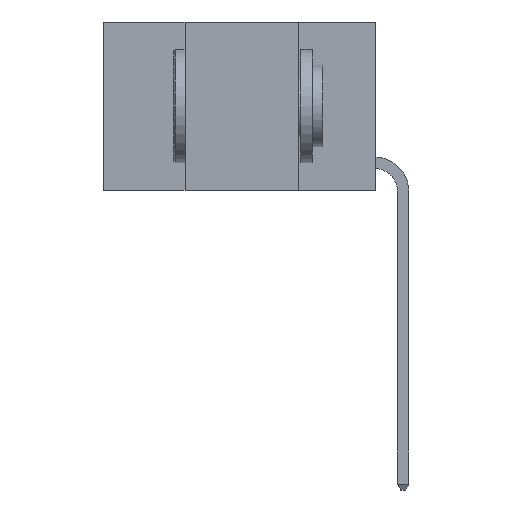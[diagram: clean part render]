
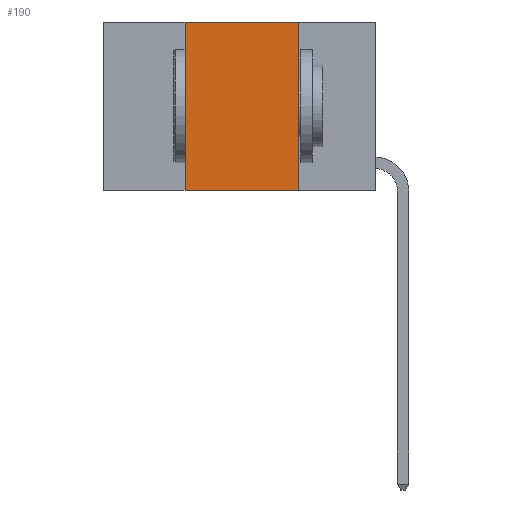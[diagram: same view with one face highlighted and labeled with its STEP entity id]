
A CAD part, left-side view. The second image highlights one B-rep face of the part: STEP entity #190.
In plain terms, the highlighted planar face has unit normal (-1, 0, 0).
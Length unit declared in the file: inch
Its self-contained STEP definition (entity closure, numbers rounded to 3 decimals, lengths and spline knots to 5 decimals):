
#190 = ADVANCED_FACE ( 'NONE', ( #4583 ), #807, .F. ) ;
#435 = CARTESIAN_POINT ( 'NONE',  ( 0., 0.42, -0.37 ) ) ;
#551 = ORIENTED_EDGE ( 'NONE', *, *, #1379, .F. ) ;
#807 = PLANE ( 'NONE',  #5528 ) ;
#838 = ORIENTED_EDGE ( 'NONE', *, *, #8155, .F. ) ;
#1355 = LINE ( 'NONE', #10478, #5852 ) ;
#1379 = EDGE_CURVE ( 'NONE', #9485, #5882, #5469, .T. ) ;
#1880 = CARTESIAN_POINT ( 'NONE',  ( 0., 0.6, 0. ) ) ;
#1991 = EDGE_CURVE ( 'NONE', #10167, #2492, #1355, .T. ) ;
#2492 = VERTEX_POINT ( 'NONE', #7672 ) ;
#3463 = DIRECTION ( 'NONE',  ( 0., 0., 1. ) ) ;
#4343 = DIRECTION ( 'NONE',  ( 0., 0., -1. ) ) ;
#4521 = ORIENTED_EDGE ( 'NONE', *, *, #6401, .T. ) ;
#4583 = FACE_OUTER_BOUND ( 'NONE', #9444, .T. ) ;
#5197 = CARTESIAN_POINT ( 'NONE',  ( 0., 0.42, 0. ) ) ;
#5469 = LINE ( 'NONE', #5197, #9484 ) ;
#5505 = LINE ( 'NONE', #11246, #7529 ) ;
#5528 = AXIS2_PLACEMENT_3D ( 'NONE', #5566, #11139, #4343 ) ;
#5566 = CARTESIAN_POINT ( 'NONE',  ( 0., 0.6, 0. ) ) ;
#5852 = VECTOR ( 'NONE', #6201, 39.37008 ) ;
#5869 = LINE ( 'NONE', #1880, #8170 ) ;
#5882 = VERTEX_POINT ( 'NONE', #8837 ) ;
#6107 = DIRECTION ( 'NONE',  ( 0., -1., 0. ) ) ;
#6201 = DIRECTION ( 'NONE',  ( 0., 0., -1. ) ) ;
#6401 = EDGE_CURVE ( 'NONE', #9485, #2492, #5505, .T. ) ;
#7529 = VECTOR ( 'NONE', #6107, 39.37008 ) ;
#7672 = CARTESIAN_POINT ( 'NONE',  ( 0., 0.17, -0.37 ) ) ;
#8155 = EDGE_CURVE ( 'NONE', #5882, #10167, #5869, .T. ) ;
#8170 = VECTOR ( 'NONE', #8928, 39.37008 ) ;
#8837 = CARTESIAN_POINT ( 'NONE',  ( 0., 0.42, 0. ) ) ;
#8928 = DIRECTION ( 'NONE',  ( 0., -1., 0. ) ) ;
#9001 = CARTESIAN_POINT ( 'NONE',  ( 0., 0.17, 0. ) ) ;
#9444 = EDGE_LOOP ( 'NONE', ( #10826, #838, #551, #4521 ) ) ;
#9484 = VECTOR ( 'NONE', #3463, 39.37008 ) ;
#9485 = VERTEX_POINT ( 'NONE', #435 ) ;
#10167 = VERTEX_POINT ( 'NONE', #9001 ) ;
#10478 = CARTESIAN_POINT ( 'NONE',  ( 0., 0.17, 0. ) ) ;
#10826 = ORIENTED_EDGE ( 'NONE', *, *, #1991, .F. ) ;
#11139 = DIRECTION ( 'NONE',  ( 1., 0., 0. ) ) ;
#11246 = CARTESIAN_POINT ( 'NONE',  ( 0., 0.6, -0.37 ) ) ;
